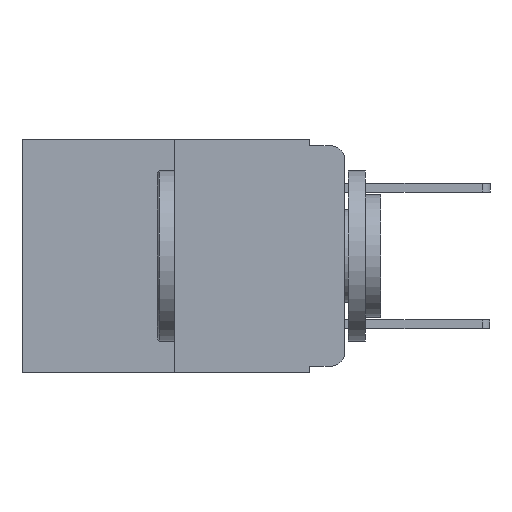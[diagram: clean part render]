
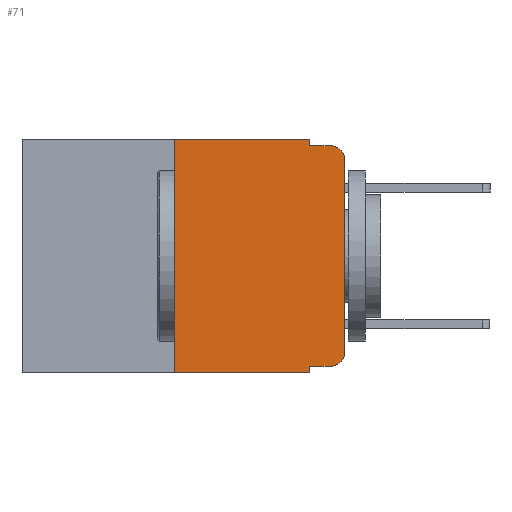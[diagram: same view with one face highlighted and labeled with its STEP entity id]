
A CAD part, left-side view. The second image highlights one B-rep face of the part: STEP entity #71.
In plain terms, the highlighted planar face has unit normal (-1, 0, 0).
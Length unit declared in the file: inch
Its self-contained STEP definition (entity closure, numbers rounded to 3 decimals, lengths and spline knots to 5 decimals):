
#71 = ADVANCED_FACE ( 'NONE', ( #1116 ), #17815, .F. ) ;
#423 = EDGE_LOOP ( 'NONE', ( #15716, #20374, #4863, #5381, #5602, #14708, #19862, #17658, #7677, #13021 ) ) ;
#468 = VERTEX_POINT ( 'NONE', #1658 ) ;
#478 = LINE ( 'NONE', #19342, #21077 ) ;
#789 = DIRECTION ( 'NONE',  ( 0., -1., 0. ) ) ;
#973 = AXIS2_PLACEMENT_3D ( 'NONE', #9274, #17748, #6008 ) ;
#1116 = FACE_OUTER_BOUND ( 'NONE', #423, .T. ) ;
#1387 = LINE ( 'NONE', #16843, #18215 ) ;
#1658 = CARTESIAN_POINT ( 'NONE',  ( 0., 0.051, -0.343 ) ) ;
#2136 = LINE ( 'NONE', #9984, #14677 ) ;
#2684 = DIRECTION ( 'NONE',  ( 0., 0., 1. ) ) ;
#3937 = EDGE_CURVE ( 'NONE', #19733, #17580, #16322, .T. ) ;
#4322 = CARTESIAN_POINT ( 'NONE',  ( 0., 0.051, 0. ) ) ;
#4463 = LINE ( 'NONE', #9243, #8337 ) ;
#4863 = ORIENTED_EDGE ( 'NONE', *, *, #10578, .F. ) ;
#4899 = VECTOR ( 'NONE', #10429, 39.37008 ) ;
#5381 = ORIENTED_EDGE ( 'NONE', *, *, #9477, .F. ) ;
#5602 = ORIENTED_EDGE ( 'NONE', *, *, #10443, .F. ) ;
#5664 = VECTOR ( 'NONE', #2684, 39.37008 ) ;
#6008 = DIRECTION ( 'NONE',  ( 0., 0., -1. ) ) ;
#6012 = VECTOR ( 'NONE', #15353, 39.37008 ) ;
#6047 = VECTOR ( 'NONE', #10936, 39.37008 ) ;
#6153 = EDGE_CURVE ( 'NONE', #11740, #19733, #17716, .T. ) ;
#6172 = LINE ( 'NONE', #18857, #5664 ) ;
#6536 = VERTEX_POINT ( 'NONE', #12993 ) ;
#7014 = DIRECTION ( 'NONE',  ( -1., 0., 0. ) ) ;
#7240 = EDGE_CURVE ( 'NONE', #11740, #468, #478, .T. ) ;
#7250 = DIRECTION ( 'NONE',  ( 0., -1., 0. ) ) ;
#7373 = CARTESIAN_POINT ( 'NONE',  ( 0., 0.051, -0.01 ) ) ;
#7677 = ORIENTED_EDGE ( 'NONE', *, *, #6153, .T. ) ;
#8036 = CARTESIAN_POINT ( 'NONE',  ( 0., 0.051, 0. ) ) ;
#8154 = DIRECTION ( 'NONE',  ( 0., 0., -1. ) ) ;
#8337 = VECTOR ( 'NONE', #789, 39.37008 ) ;
#8373 = EDGE_CURVE ( 'NONE', #6536, #10029, #2136, .T. ) ;
#9243 = CARTESIAN_POINT ( 'NONE',  ( 0., 0.051, -0.01 ) ) ;
#9274 = CARTESIAN_POINT ( 'NONE',  ( 0., 0.473, 0. ) ) ;
#9385 = DIRECTION ( 'NONE',  ( -1., 0., 0. ) ) ;
#9477 = EDGE_CURVE ( 'NONE', #19729, #19461, #10430, .T. ) ;
#9984 = CARTESIAN_POINT ( 'NONE',  ( 0., 0.25, 0. ) ) ;
#9999 = CARTESIAN_POINT ( 'NONE',  ( 0., 0., -0.313 ) ) ;
#10029 = VERTEX_POINT ( 'NONE', #10563 ) ;
#10053 = DIRECTION ( 'NONE',  ( 0., 0., 1. ) ) ;
#10396 = LINE ( 'NONE', #13793, #6012 ) ;
#10429 = DIRECTION ( 'NONE',  ( 0., -1., 0. ) ) ;
#10430 = LINE ( 'NONE', #4322, #6047 ) ;
#10443 = EDGE_CURVE ( 'NONE', #10029, #19729, #10396, .T. ) ;
#10563 = CARTESIAN_POINT ( 'NONE',  ( 0., 0.25, 0. ) ) ;
#10578 = EDGE_CURVE ( 'NONE', #19461, #18821, #4463, .T. ) ;
#10936 = DIRECTION ( 'NONE',  ( 0., 0., -1. ) ) ;
#11165 = VERTEX_POINT ( 'NONE', #19993 ) ;
#11643 = EDGE_CURVE ( 'NONE', #11165, #18821, #15786, .T. ) ;
#11740 = VERTEX_POINT ( 'NONE', #15245 ) ;
#12701 = EDGE_CURVE ( 'NONE', #17580, #11165, #6172, .T. ) ;
#12993 = CARTESIAN_POINT ( 'NONE',  ( 0., 0.25, -0.343 ) ) ;
#13021 = ORIENTED_EDGE ( 'NONE', *, *, #3937, .T. ) ;
#13145 = AXIS2_PLACEMENT_3D ( 'NONE', #16611, #7014, #18198 ) ;
#13793 = CARTESIAN_POINT ( 'NONE',  ( 0., 0.473, 0. ) ) ;
#14677 = VECTOR ( 'NONE', #10053, 39.37008 ) ;
#14708 = ORIENTED_EDGE ( 'NONE', *, *, #8373, .F. ) ;
#15245 = CARTESIAN_POINT ( 'NONE',  ( 0., 0.051, -0.333 ) ) ;
#15353 = DIRECTION ( 'NONE',  ( 0., -1., 0. ) ) ;
#15473 = EDGE_CURVE ( 'NONE', #6536, #468, #1387, .T. ) ;
#15716 = ORIENTED_EDGE ( 'NONE', *, *, #12701, .T. ) ;
#15786 = CIRCLE ( 'NONE', #13145, 0.02 ) ;
#16322 = CIRCLE ( 'NONE', #19382, 0.02 ) ;
#16611 = CARTESIAN_POINT ( 'NONE',  ( 0., 0.02, -0.03 ) ) ;
#16843 = CARTESIAN_POINT ( 'NONE',  ( 0., 0.473, -0.343 ) ) ;
#17501 = CARTESIAN_POINT ( 'NONE',  ( 0., 0.02, -0.333 ) ) ;
#17580 = VERTEX_POINT ( 'NONE', #9999 ) ;
#17658 = ORIENTED_EDGE ( 'NONE', *, *, #7240, .F. ) ;
#17716 = LINE ( 'NONE', #18284, #4899 ) ;
#17748 = DIRECTION ( 'NONE',  ( 1., 0., 0. ) ) ;
#17815 = PLANE ( 'NONE',  #973 ) ;
#18198 = DIRECTION ( 'NONE',  ( 0., 0., -1. ) ) ;
#18215 = VECTOR ( 'NONE', #7250, 39.37008 ) ;
#18284 = CARTESIAN_POINT ( 'NONE',  ( 0., 0.051, -0.333 ) ) ;
#18713 = CARTESIAN_POINT ( 'NONE',  ( 0., 0.02, -0.01 ) ) ;
#18821 = VERTEX_POINT ( 'NONE', #18713 ) ;
#18857 = CARTESIAN_POINT ( 'NONE',  ( 0., 0., 0. ) ) ;
#18866 = CARTESIAN_POINT ( 'NONE',  ( 0., 0.02, -0.313 ) ) ;
#19342 = CARTESIAN_POINT ( 'NONE',  ( 0., 0.051, 0. ) ) ;
#19382 = AXIS2_PLACEMENT_3D ( 'NONE', #18866, #9385, #20434 ) ;
#19461 = VERTEX_POINT ( 'NONE', #7373 ) ;
#19729 = VERTEX_POINT ( 'NONE', #8036 ) ;
#19733 = VERTEX_POINT ( 'NONE', #17501 ) ;
#19862 = ORIENTED_EDGE ( 'NONE', *, *, #15473, .T. ) ;
#19993 = CARTESIAN_POINT ( 'NONE',  ( 0., 0., -0.03 ) ) ;
#20374 = ORIENTED_EDGE ( 'NONE', *, *, #11643, .T. ) ;
#20434 = DIRECTION ( 'NONE',  ( 0., 0., -1. ) ) ;
#21077 = VECTOR ( 'NONE', #8154, 39.37008 ) ;
